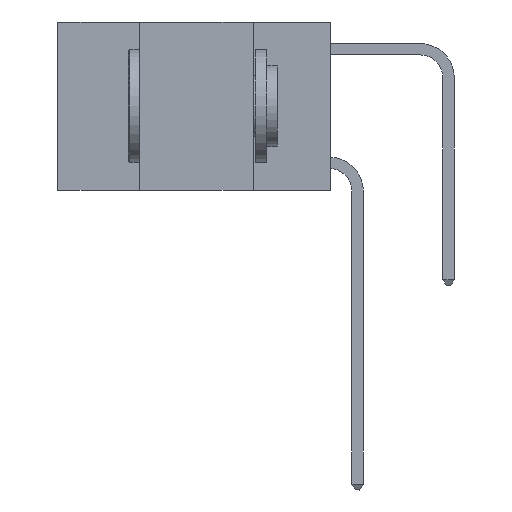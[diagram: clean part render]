
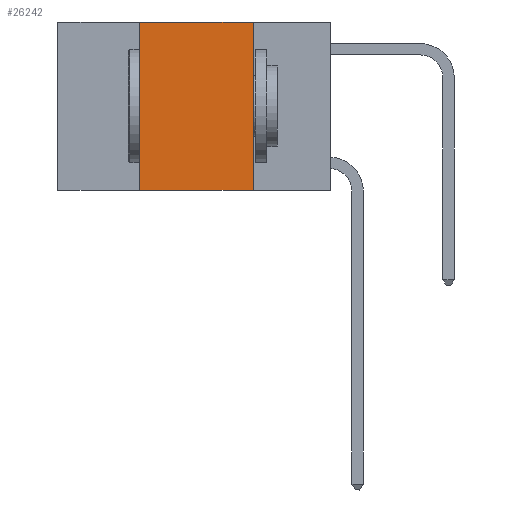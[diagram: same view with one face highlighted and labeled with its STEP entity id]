
A CAD part, left-side view. The second image highlights one B-rep face of the part: STEP entity #26242.
In plain terms, the highlighted planar face has unit normal (-1, 0, 0).
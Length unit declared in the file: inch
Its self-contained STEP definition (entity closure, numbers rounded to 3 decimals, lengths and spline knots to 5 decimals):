
#1448 = VERTEX_POINT ( 'NONE', #10307 ) ;
#1472 = CARTESIAN_POINT ( 'NONE',  ( 0., 0.17, 0. ) ) ;
#2264 = CARTESIAN_POINT ( 'NONE',  ( 0., 0.42, 0. ) ) ;
#2709 = LINE ( 'NONE', #1472, #26098 ) ;
#4421 = CARTESIAN_POINT ( 'NONE',  ( 0., 0.6, 0. ) ) ;
#5452 = CARTESIAN_POINT ( 'NONE',  ( 0., 0.17, -0.37 ) ) ;
#5574 = VECTOR ( 'NONE', #23903, 39.37008 ) ;
#7480 = PLANE ( 'NONE',  #10503 ) ;
#7620 = EDGE_CURVE ( 'NONE', #1448, #23316, #25782, .T. ) ;
#8043 = CARTESIAN_POINT ( 'NONE',  ( 0., 0.17, 0. ) ) ;
#8045 = CARTESIAN_POINT ( 'NONE',  ( 0., 0.42, 0. ) ) ;
#9540 = CARTESIAN_POINT ( 'NONE',  ( 0., 0.6, 0. ) ) ;
#9672 = VECTOR ( 'NONE', #20977, 39.37008 ) ;
#9770 = DIRECTION ( 'NONE',  ( 0., 0., -1. ) ) ;
#10307 = CARTESIAN_POINT ( 'NONE',  ( 0., 0.42, -0.37 ) ) ;
#10503 = AXIS2_PLACEMENT_3D ( 'NONE', #9540, #11637, #26134 ) ;
#10525 = VECTOR ( 'NONE', #20513, 39.37008 ) ;
#11637 = DIRECTION ( 'NONE',  ( 1., 0., 0. ) ) ;
#11869 = ORIENTED_EDGE ( 'NONE', *, *, #21570, .F. ) ;
#12498 = ORIENTED_EDGE ( 'NONE', *, *, #23456, .T. ) ;
#16570 = LINE ( 'NONE', #21841, #5574 ) ;
#18398 = EDGE_LOOP ( 'NONE', ( #11869, #22126, #23579, #12498 ) ) ;
#19134 = EDGE_CURVE ( 'NONE', #23316, #24365, #26227, .T. ) ;
#20513 = DIRECTION ( 'NONE',  ( 0., 0., 1. ) ) ;
#20977 = DIRECTION ( 'NONE',  ( 0., -1., 0. ) ) ;
#21570 = EDGE_CURVE ( 'NONE', #24365, #24181, #2709, .T. ) ;
#21841 = CARTESIAN_POINT ( 'NONE',  ( 0., 0.6, -0.37 ) ) ;
#22126 = ORIENTED_EDGE ( 'NONE', *, *, #19134, .F. ) ;
#23316 = VERTEX_POINT ( 'NONE', #2264 ) ;
#23456 = EDGE_CURVE ( 'NONE', #1448, #24181, #16570, .T. ) ;
#23579 = ORIENTED_EDGE ( 'NONE', *, *, #7620, .F. ) ;
#23903 = DIRECTION ( 'NONE',  ( 0., -1., 0. ) ) ;
#24181 = VERTEX_POINT ( 'NONE', #5452 ) ;
#24365 = VERTEX_POINT ( 'NONE', #8043 ) ;
#25325 = FACE_OUTER_BOUND ( 'NONE', #18398, .T. ) ;
#25782 = LINE ( 'NONE', #8045, #10525 ) ;
#26098 = VECTOR ( 'NONE', #9770, 39.37008 ) ;
#26134 = DIRECTION ( 'NONE',  ( 0., 0., -1. ) ) ;
#26227 = LINE ( 'NONE', #4421, #9672 ) ;
#26242 = ADVANCED_FACE ( 'NONE', ( #25325 ), #7480, .F. ) ;
